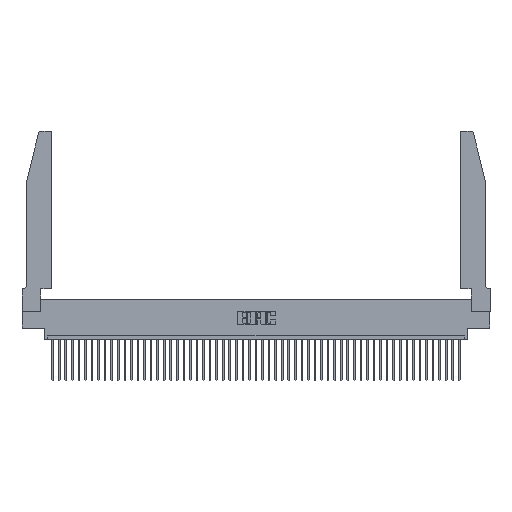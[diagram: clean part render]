
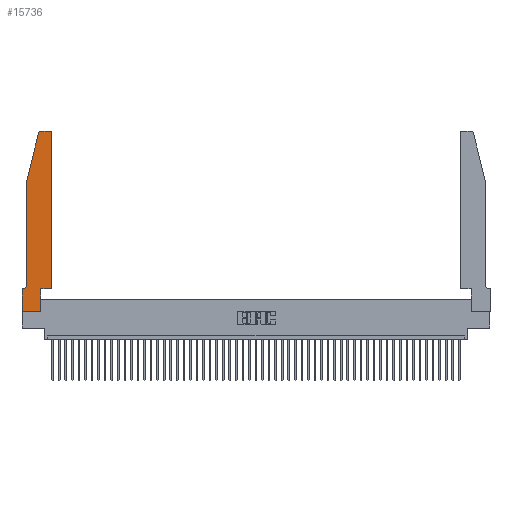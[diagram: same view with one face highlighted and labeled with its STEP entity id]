
A CAD part, top view. The second image highlights one B-rep face of the part: STEP entity #15736.
In plain terms, the highlighted planar face has unit normal (0, 0, 1).
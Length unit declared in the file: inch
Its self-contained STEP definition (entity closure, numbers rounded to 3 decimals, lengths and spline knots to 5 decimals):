
#225 = EDGE_CURVE ( 'NONE', #1987, #43029, #40246, .T. ) ;
#1302 = EDGE_CURVE ( 'NONE', #42258, #1987, #13702, .T. ) ;
#1987 = VERTEX_POINT ( 'NONE', #45834 ) ;
#2143 = VERTEX_POINT ( 'NONE', #28754 ) ;
#2757 = VERTEX_POINT ( 'NONE', #25094 ) ;
#3557 = LINE ( 'NONE', #46409, #42484 ) ;
#5334 = EDGE_CURVE ( 'NONE', #35715, #30850, #44755, .T. ) ;
#5715 = EDGE_CURVE ( 'NONE', #13380, #23154, #30422, .T. ) ;
#6417 = CARTESIAN_POINT ( 'NONE',  ( 0.0755, 2., 0.37 ) ) ;
#6460 = ORIENTED_EDGE ( 'NONE', *, *, #27116, .T. ) ;
#6525 = CARTESIAN_POINT ( 'NONE',  ( 0.4505, 0.35, 0.37 ) ) ;
#7497 = ORIENTED_EDGE ( 'NONE', *, *, #225, .T. ) ;
#7940 = ORIENTED_EDGE ( 'NONE', *, *, #21247, .T. ) ;
#8504 = EDGE_CURVE ( 'NONE', #43029, #2143, #47287, .T. ) ;
#9249 = CARTESIAN_POINT ( 'NONE',  ( 0., 0., 0.37 ) ) ;
#10448 = CARTESIAN_POINT ( 'NONE',  ( 0.4205, 2.72, 0.37 ) ) ;
#10576 = DIRECTION ( 'NONE',  ( 1., 0., 0. ) ) ;
#11385 = EDGE_CURVE ( 'NONE', #30850, #2757, #19440, .T. ) ;
#12144 = CARTESIAN_POINT ( 'NONE',  ( 0.0055, 0.42, 0.37 ) ) ;
#12511 = DIRECTION ( 'NONE',  ( 0., 1., 0. ) ) ;
#12847 = LINE ( 'NONE', #6417, #32117 ) ;
#13380 = VERTEX_POINT ( 'NONE', #33324 ) ;
#13471 = ORIENTED_EDGE ( 'NONE', *, *, #11385, .T. ) ;
#13702 = CIRCLE ( 'NONE', #19914, 0.03 ) ;
#13965 = EDGE_LOOP ( 'NONE', ( #7497, #36078, #27554, #39921, #13471, #27840, #6460, #7940, #15926, #31756, #28643, #49269 ) ) ;
#14631 = CARTESIAN_POINT ( 'NONE',  ( 0.4505, 2.72, 0.37 ) ) ;
#15736 = ADVANCED_FACE ( 'NONE', ( #18845 ), #40439, .T. ) ;
#15926 = ORIENTED_EDGE ( 'NONE', *, *, #5715, .T. ) ;
#16158 = DIRECTION ( 'NONE',  ( -1., 0., 0. ) ) ;
#17759 = CARTESIAN_POINT ( 'NONE',  ( 0., 0.35, 0.37 ) ) ;
#17971 = CARTESIAN_POINT ( 'NONE',  ( 0.0755, 2., 0.37 ) ) ;
#18129 = CARTESIAN_POINT ( 'NONE',  ( 0., 0.35, 0.37 ) ) ;
#18221 = CARTESIAN_POINT ( 'NONE',  ( 0.2865, 0.35, 0.37 ) ) ;
#18845 = FACE_OUTER_BOUND ( 'NONE', #13965, .T. ) ;
#19104 = EDGE_CURVE ( 'NONE', #26157, #42258, #3557, .T. ) ;
#19440 = CIRCLE ( 'NONE', #36011, 0.07 ) ;
#19835 = DIRECTION ( 'NONE',  ( 0., -1., 0. ) ) ;
#19914 = AXIS2_PLACEMENT_3D ( 'NONE', #10448, #37326, #37640 ) ;
#20168 = CARTESIAN_POINT ( 'NONE',  ( 0., 0., 0.37 ) ) ;
#21205 = CARTESIAN_POINT ( 'NONE',  ( 0.0755, 2., 0.37 ) ) ;
#21247 = EDGE_CURVE ( 'NONE', #45995, #13380, #32030, .T. ) ;
#21984 = LINE ( 'NONE', #47493, #37608 ) ;
#22867 = CARTESIAN_POINT ( 'NONE',  ( 0.4505, 0.35, 0.37 ) ) ;
#23154 = VERTEX_POINT ( 'NONE', #33091 ) ;
#23325 = EDGE_CURVE ( 'NONE', #2143, #35715, #12847, .T. ) ;
#24274 = DIRECTION ( 'NONE',  ( -1., 0., 0. ) ) ;
#25094 = CARTESIAN_POINT ( 'NONE',  ( 0.0055, 0.35, 0.37 ) ) ;
#26157 = VERTEX_POINT ( 'NONE', #6525 ) ;
#27116 = EDGE_CURVE ( 'NONE', #40820, #45995, #32273, .T. ) ;
#27554 = ORIENTED_EDGE ( 'NONE', *, *, #23325, .T. ) ;
#27599 = VECTOR ( 'NONE', #42220, 39.37008 ) ;
#27840 = ORIENTED_EDGE ( 'NONE', *, *, #29817, .T. ) ;
#27905 = VECTOR ( 'NONE', #33359, 39.37008 ) ;
#28581 = DIRECTION ( 'NONE',  ( 1., 0., 0. ) ) ;
#28643 = ORIENTED_EDGE ( 'NONE', *, *, #19104, .T. ) ;
#28754 = CARTESIAN_POINT ( 'NONE',  ( 0.25487, 2.72718, 0.37 ) ) ;
#28789 = VECTOR ( 'NONE', #38763, 39.37008 ) ;
#29095 = DIRECTION ( 'NONE',  ( 0., 0., 1. ) ) ;
#29817 = EDGE_CURVE ( 'NONE', #2757, #40820, #21984, .T. ) ;
#30422 = LINE ( 'NONE', #18221, #27905 ) ;
#30850 = VERTEX_POINT ( 'NONE', #41249 ) ;
#31756 = ORIENTED_EDGE ( 'NONE', *, *, #42917, .T. ) ;
#32030 = LINE ( 'NONE', #9249, #43360 ) ;
#32117 = VECTOR ( 'NONE', #48061, 39.37008 ) ;
#32273 = LINE ( 'NONE', #20168, #45418 ) ;
#32407 = AXIS2_PLACEMENT_3D ( 'NONE', #43756, #29095, #36490 ) ;
#33091 = CARTESIAN_POINT ( 'NONE',  ( 0.2865, 0.35, 0.37 ) ) ;
#33324 = CARTESIAN_POINT ( 'NONE',  ( 0.2865, 0., 0.37 ) ) ;
#33359 = DIRECTION ( 'NONE',  ( 0., 1., 0. ) ) ;
#33930 = AXIS2_PLACEMENT_3D ( 'NONE', #18129, #48713, #10576 ) ;
#35114 = CARTESIAN_POINT ( 'NONE',  ( 0.284, 2.75, 0.37 ) ) ;
#35715 = VERTEX_POINT ( 'NONE', #21205 ) ;
#36011 = AXIS2_PLACEMENT_3D ( 'NONE', #12144, #44018, #16158 ) ;
#36078 = ORIENTED_EDGE ( 'NONE', *, *, #8504, .T. ) ;
#36490 = DIRECTION ( 'NONE',  ( 1., 0., 0. ) ) ;
#37326 = DIRECTION ( 'NONE',  ( 0., 0., 1. ) ) ;
#37608 = VECTOR ( 'NONE', #24274, 39.37008 ) ;
#37640 = DIRECTION ( 'NONE',  ( 1., 0., 0. ) ) ;
#38537 = CARTESIAN_POINT ( 'NONE',  ( 0.2605, 2.75, 0.37 ) ) ;
#38763 = DIRECTION ( 'NONE',  ( 1., 0., 0. ) ) ;
#39354 = VECTOR ( 'NONE', #44938, 39.37008 ) ;
#39921 = ORIENTED_EDGE ( 'NONE', *, *, #5334, .T. ) ;
#40246 = LINE ( 'NONE', #38537, #27599 ) ;
#40439 = PLANE ( 'NONE',  #33930 ) ;
#40820 = VERTEX_POINT ( 'NONE', #17759 ) ;
#40833 = LINE ( 'NONE', #22867, #28789 ) ;
#41249 = CARTESIAN_POINT ( 'NONE',  ( 0.0755, 0.42, 0.37 ) ) ;
#42220 = DIRECTION ( 'NONE',  ( -1., 0., 0. ) ) ;
#42258 = VERTEX_POINT ( 'NONE', #14631 ) ;
#42484 = VECTOR ( 'NONE', #12511, 39.37008 ) ;
#42917 = EDGE_CURVE ( 'NONE', #23154, #26157, #40833, .T. ) ;
#43029 = VERTEX_POINT ( 'NONE', #35114 ) ;
#43360 = VECTOR ( 'NONE', #28581, 39.37008 ) ;
#43756 = CARTESIAN_POINT ( 'NONE',  ( 0.284, 2.72, 0.37 ) ) ;
#44018 = DIRECTION ( 'NONE',  ( 0., 0., -1. ) ) ;
#44755 = LINE ( 'NONE', #17971, #39354 ) ;
#44938 = DIRECTION ( 'NONE',  ( 0., -1., 0. ) ) ;
#45418 = VECTOR ( 'NONE', #19835, 39.37008 ) ;
#45834 = CARTESIAN_POINT ( 'NONE',  ( 0.4205, 2.75, 0.37 ) ) ;
#45995 = VERTEX_POINT ( 'NONE', #48143 ) ;
#46409 = CARTESIAN_POINT ( 'NONE',  ( 0.4505, 0.35, 0.37 ) ) ;
#47287 = CIRCLE ( 'NONE', #32407, 0.03 ) ;
#47493 = CARTESIAN_POINT ( 'NONE',  ( 0.0755, 0.35, 0.37 ) ) ;
#48061 = DIRECTION ( 'NONE',  ( -0.239, -0.971, 0. ) ) ;
#48143 = CARTESIAN_POINT ( 'NONE',  ( 0., 0., 0.37 ) ) ;
#48713 = DIRECTION ( 'NONE',  ( 0., 0., 1. ) ) ;
#49269 = ORIENTED_EDGE ( 'NONE', *, *, #1302, .T. ) ;
